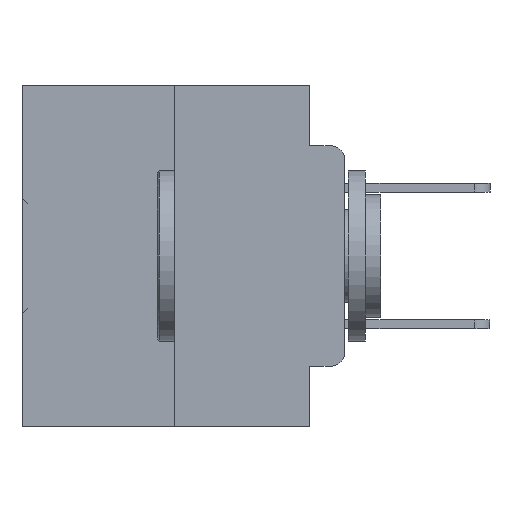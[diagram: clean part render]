
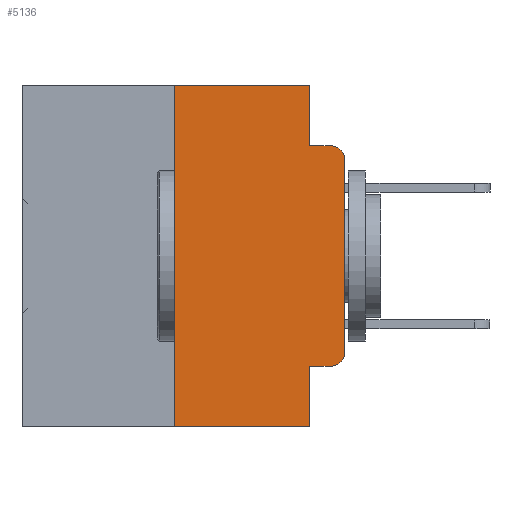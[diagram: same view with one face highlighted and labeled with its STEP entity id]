
A CAD part, left-side view. The second image highlights one B-rep face of the part: STEP entity #5136.
In plain terms, the highlighted planar face has unit normal (-1, 0, 0).
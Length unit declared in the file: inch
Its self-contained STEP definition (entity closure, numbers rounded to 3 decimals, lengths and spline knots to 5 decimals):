
#374 = EDGE_CURVE ( 'NONE', #6044, #5016, #1457, .T. ) ;
#418 = VECTOR ( 'NONE', #25328, 39.37008 ) ;
#1457 = LINE ( 'NONE', #21067, #23505 ) ;
#2922 = DIRECTION ( 'NONE',  ( -1., 0., 0. ) ) ;
#3266 = EDGE_CURVE ( 'NONE', #28123, #25981, #29700, .T. ) ;
#3279 = VECTOR ( 'NONE', #23416, 39.37008 ) ;
#3283 = ORIENTED_EDGE ( 'NONE', *, *, #374, .F. ) ;
#3515 = ORIENTED_EDGE ( 'NONE', *, *, #25905, .F. ) ;
#3755 = EDGE_CURVE ( 'NONE', #25019, #11743, #22430, .T. ) ;
#4156 = CARTESIAN_POINT ( 'NONE',  ( 0., 0.051, -0.4115 ) ) ;
#4226 = CARTESIAN_POINT ( 'NONE',  ( 0., 0.25, -0.5 ) ) ;
#5016 = VERTEX_POINT ( 'NONE', #28015 ) ;
#5136 = ADVANCED_FACE ( 'NONE', ( #23903 ), #20369, .F. ) ;
#5952 = VERTEX_POINT ( 'NONE', #23764 ) ;
#5986 = CARTESIAN_POINT ( 'NONE',  ( 0., 0.473, -0.5 ) ) ;
#6044 = VERTEX_POINT ( 'NONE', #18762 ) ;
#6650 = CARTESIAN_POINT ( 'NONE',  ( 0., 0.051, -0.4115 ) ) ;
#6683 = CARTESIAN_POINT ( 'NONE',  ( 0., 0.473, 0. ) ) ;
#7970 = LINE ( 'NONE', #28173, #418 ) ;
#8774 = ORIENTED_EDGE ( 'NONE', *, *, #3266, .F. ) ;
#8827 = DIRECTION ( 'NONE',  ( 0., -1., 0. ) ) ;
#9497 = DIRECTION ( 'NONE',  ( 1., 0., 0. ) ) ;
#11412 = CARTESIAN_POINT ( 'NONE',  ( 0., 0.051, -0.0885 ) ) ;
#11426 = VECTOR ( 'NONE', #8827, 39.37008 ) ;
#11626 = ORIENTED_EDGE ( 'NONE', *, *, #31153, .F. ) ;
#11743 = VERTEX_POINT ( 'NONE', #18822 ) ;
#12193 = VECTOR ( 'NONE', #14806, 39.37008 ) ;
#12735 = CARTESIAN_POINT ( 'NONE',  ( 0., 0.02, -0.1085 ) ) ;
#13049 = VERTEX_POINT ( 'NONE', #4226 ) ;
#13470 = ORIENTED_EDGE ( 'NONE', *, *, #14238, .T. ) ;
#13559 = VERTEX_POINT ( 'NONE', #20124 ) ;
#13904 = LINE ( 'NONE', #31137, #12193 ) ;
#14215 = ORIENTED_EDGE ( 'NONE', *, *, #26117, .T. ) ;
#14238 = EDGE_CURVE ( 'NONE', #17500, #25019, #25288, .T. ) ;
#14806 = DIRECTION ( 'NONE',  ( 0., 0., -1. ) ) ;
#15217 = VECTOR ( 'NONE', #20120, 39.37008 ) ;
#15484 = DIRECTION ( 'NONE',  ( 0., 0., -1. ) ) ;
#15819 = CARTESIAN_POINT ( 'NONE',  ( 0., 0.02, -0.4115 ) ) ;
#17049 = DIRECTION ( 'NONE',  ( 0., -1., 0. ) ) ;
#17500 = VERTEX_POINT ( 'NONE', #6650 ) ;
#18638 = ORIENTED_EDGE ( 'NONE', *, *, #32721, .T. ) ;
#18762 = CARTESIAN_POINT ( 'NONE',  ( 0., 0.25, 0. ) ) ;
#18822 = CARTESIAN_POINT ( 'NONE',  ( 0., 0., -0.3915 ) ) ;
#18899 = EDGE_LOOP ( 'NONE', ( #14215, #18638, #8774, #11626, #3283, #25099, #23328, #3515, #13470, #29774 ) ) ;
#18924 = CIRCLE ( 'NONE', #24641, 0.02 ) ;
#19024 = VECTOR ( 'NONE', #26616, 39.37008 ) ;
#19519 = CARTESIAN_POINT ( 'NONE',  ( 0., 0.02, -0.3915 ) ) ;
#20120 = DIRECTION ( 'NONE',  ( 0., -1., 0. ) ) ;
#20124 = CARTESIAN_POINT ( 'NONE',  ( 0., 0.051, -0.5 ) ) ;
#20369 = PLANE ( 'NONE',  #28915 ) ;
#21067 = CARTESIAN_POINT ( 'NONE',  ( 0., 0.473, 0. ) ) ;
#21099 = DIRECTION ( 'NONE',  ( 0., 0., 1. ) ) ;
#21100 = CARTESIAN_POINT ( 'NONE',  ( 0., 0.25, 0. ) ) ;
#22066 = VECTOR ( 'NONE', #21099, 39.37008 ) ;
#22237 = DIRECTION ( 'NONE',  ( 0., 0., -1. ) ) ;
#22430 = CIRCLE ( 'NONE', #29999, 0.02 ) ;
#23328 = ORIENTED_EDGE ( 'NONE', *, *, #25807, .T. ) ;
#23416 = DIRECTION ( 'NONE',  ( 0., -1., 0. ) ) ;
#23505 = VECTOR ( 'NONE', #17049, 39.37008 ) ;
#23764 = CARTESIAN_POINT ( 'NONE',  ( 0., 0., -0.1085 ) ) ;
#23903 = FACE_OUTER_BOUND ( 'NONE', #18899, .T. ) ;
#24641 = AXIS2_PLACEMENT_3D ( 'NONE', #12735, #31812, #15484 ) ;
#25019 = VERTEX_POINT ( 'NONE', #15819 ) ;
#25099 = ORIENTED_EDGE ( 'NONE', *, *, #31363, .F. ) ;
#25288 = LINE ( 'NONE', #4156, #3279 ) ;
#25328 = DIRECTION ( 'NONE',  ( 0., 0., -1. ) ) ;
#25512 = CARTESIAN_POINT ( 'NONE',  ( 0., 0.051, -0.0885 ) ) ;
#25807 = EDGE_CURVE ( 'NONE', #13049, #13559, #33195, .T. ) ;
#25905 = EDGE_CURVE ( 'NONE', #17500, #13559, #7970, .T. ) ;
#25981 = VERTEX_POINT ( 'NONE', #28633 ) ;
#26117 = EDGE_CURVE ( 'NONE', #11743, #5952, #29317, .T. ) ;
#26616 = DIRECTION ( 'NONE',  ( 0., 0., 1. ) ) ;
#28015 = CARTESIAN_POINT ( 'NONE',  ( 0., 0.051, 0. ) ) ;
#28123 = VERTEX_POINT ( 'NONE', #11412 ) ;
#28173 = CARTESIAN_POINT ( 'NONE',  ( 0., 0.051, 0. ) ) ;
#28591 = DIRECTION ( 'NONE',  ( 0., 0., -1. ) ) ;
#28633 = CARTESIAN_POINT ( 'NONE',  ( 0., 0.02, -0.0885 ) ) ;
#28915 = AXIS2_PLACEMENT_3D ( 'NONE', #6683, #9497, #28591 ) ;
#29317 = LINE ( 'NONE', #31951, #22066 ) ;
#29700 = LINE ( 'NONE', #25512, #15217 ) ;
#29774 = ORIENTED_EDGE ( 'NONE', *, *, #3755, .T. ) ;
#29999 = AXIS2_PLACEMENT_3D ( 'NONE', #19519, #2922, #22237 ) ;
#31137 = CARTESIAN_POINT ( 'NONE',  ( 0., 0.051, 0. ) ) ;
#31153 = EDGE_CURVE ( 'NONE', #5016, #28123, #13904, .T. ) ;
#31363 = EDGE_CURVE ( 'NONE', #13049, #6044, #33536, .T. ) ;
#31812 = DIRECTION ( 'NONE',  ( -1., 0., 0. ) ) ;
#31951 = CARTESIAN_POINT ( 'NONE',  ( 0., 0., 0. ) ) ;
#32721 = EDGE_CURVE ( 'NONE', #5952, #25981, #18924, .T. ) ;
#33195 = LINE ( 'NONE', #5986, #11426 ) ;
#33536 = LINE ( 'NONE', #21100, #19024 ) ;
